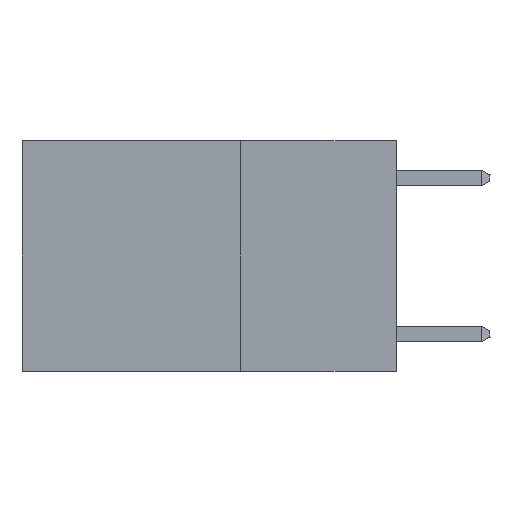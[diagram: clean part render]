
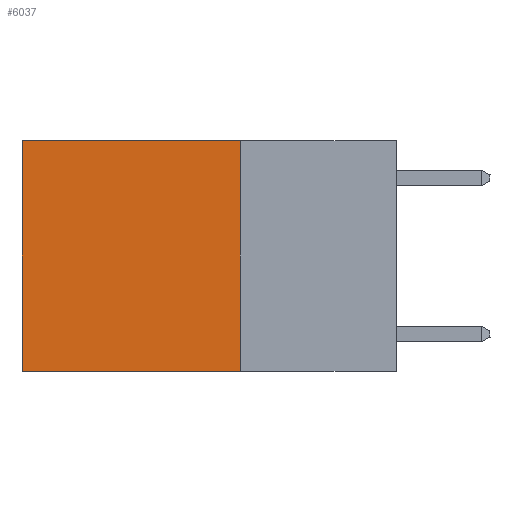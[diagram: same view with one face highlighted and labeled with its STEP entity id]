
A CAD part, left-side view. The second image highlights one B-rep face of the part: STEP entity #6037.
In plain terms, the highlighted planar face has unit normal (-1, 0, 0).
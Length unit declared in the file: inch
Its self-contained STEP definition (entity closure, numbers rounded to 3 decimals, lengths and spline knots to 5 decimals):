
#116 = CARTESIAN_POINT ( 'NONE',  ( 0.2625, 0.25, 0. ) ) ;
#673 = EDGE_CURVE ( 'NONE', #1029, #3194, #10342, .T. ) ;
#881 = CARTESIAN_POINT ( 'NONE',  ( 0.2625, 0.6, 0. ) ) ;
#1029 = VERTEX_POINT ( 'NONE', #1935 ) ;
#1079 = CARTESIAN_POINT ( 'NONE',  ( 0.2625, 0.25, -0.37 ) ) ;
#1474 = VERTEX_POINT ( 'NONE', #14805 ) ;
#1935 = CARTESIAN_POINT ( 'NONE',  ( 0.2625, 0.25, 0. ) ) ;
#2403 = VERTEX_POINT ( 'NONE', #6983 ) ;
#2787 = PLANE ( 'NONE',  #4720 ) ;
#3024 = ORIENTED_EDGE ( 'NONE', *, *, #4647, .F. ) ;
#3168 = ORIENTED_EDGE ( 'NONE', *, *, #673, .F. ) ;
#3194 = VERTEX_POINT ( 'NONE', #6601 ) ;
#3446 = VECTOR ( 'NONE', #13740, 39.37008 ) ;
#3698 = EDGE_CURVE ( 'NONE', #1029, #2403, #13881, .T. ) ;
#4352 = VECTOR ( 'NONE', #6347, 39.37008 ) ;
#4621 = DIRECTION ( 'NONE',  ( 0., 0., -1. ) ) ;
#4647 = EDGE_CURVE ( 'NONE', #3194, #1474, #11439, .T. ) ;
#4720 = AXIS2_PLACEMENT_3D ( 'NONE', #8222, #7602, #8683 ) ;
#5063 = FACE_OUTER_BOUND ( 'NONE', #9933, .T. ) ;
#6037 = ADVANCED_FACE ( 'NONE', ( #5063 ), #2787, .F. ) ;
#6347 = DIRECTION ( 'NONE',  ( 0., 0., -1. ) ) ;
#6601 = CARTESIAN_POINT ( 'NONE',  ( 0.2625, 0.25, -0.37 ) ) ;
#6852 = VECTOR ( 'NONE', #7023, 39.37008 ) ;
#6983 = CARTESIAN_POINT ( 'NONE',  ( 0.2625, 0.6, 0. ) ) ;
#7023 = DIRECTION ( 'NONE',  ( 0., 1., 0. ) ) ;
#7602 = DIRECTION ( 'NONE',  ( 1., 0., 0. ) ) ;
#8222 = CARTESIAN_POINT ( 'NONE',  ( 0.2625, 0.25, 0. ) ) ;
#8683 = DIRECTION ( 'NONE',  ( 0., 0., -1. ) ) ;
#9167 = CARTESIAN_POINT ( 'NONE',  ( 0.2625, 0.25, 0. ) ) ;
#9895 = LINE ( 'NONE', #881, #4352 ) ;
#9933 = EDGE_LOOP ( 'NONE', ( #11744, #3024, #3168, #11406 ) ) ;
#10342 = LINE ( 'NONE', #116, #13702 ) ;
#11406 = ORIENTED_EDGE ( 'NONE', *, *, #3698, .T. ) ;
#11439 = LINE ( 'NONE', #1079, #6852 ) ;
#11744 = ORIENTED_EDGE ( 'NONE', *, *, #13071, .T. ) ;
#13071 = EDGE_CURVE ( 'NONE', #2403, #1474, #9895, .T. ) ;
#13702 = VECTOR ( 'NONE', #4621, 39.37008 ) ;
#13740 = DIRECTION ( 'NONE',  ( 0., 1., 0. ) ) ;
#13881 = LINE ( 'NONE', #9167, #3446 ) ;
#14805 = CARTESIAN_POINT ( 'NONE',  ( 0.2625, 0.6, -0.37 ) ) ;
